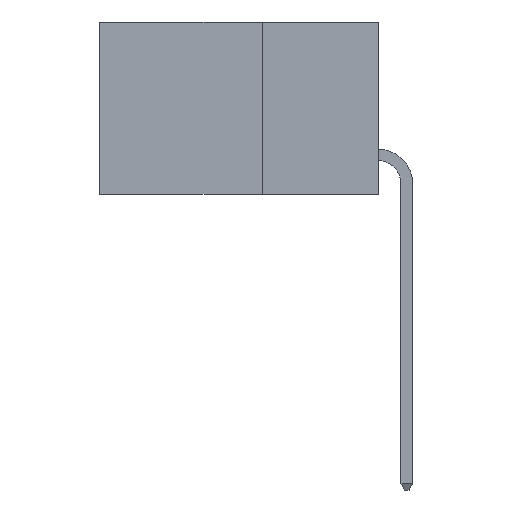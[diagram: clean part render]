
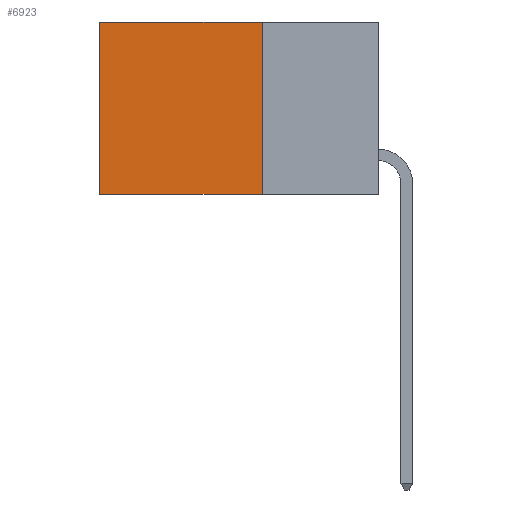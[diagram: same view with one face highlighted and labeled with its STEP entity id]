
A CAD part, left-side view. The second image highlights one B-rep face of the part: STEP entity #6923.
In plain terms, the highlighted planar face has unit normal (-1, 0, 0).
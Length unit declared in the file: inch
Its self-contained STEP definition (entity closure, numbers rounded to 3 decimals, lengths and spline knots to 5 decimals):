
#211 = CARTESIAN_POINT ( 'NONE',  ( 0.2615, 0.25, -0.37 ) ) ;
#429 = EDGE_CURVE ( 'NONE', #11617, #3420, #15281, .T. ) ;
#715 = DIRECTION ( 'NONE',  ( 0., 0., -1. ) ) ;
#1415 = EDGE_CURVE ( 'NONE', #8725, #10279, #13659, .T. ) ;
#1551 = DIRECTION ( 'NONE',  ( 0., 1., 0. ) ) ;
#1639 = DIRECTION ( 'NONE',  ( 0., 0., -1. ) ) ;
#2571 = DIRECTION ( 'NONE',  ( 0., 1., 0. ) ) ;
#2729 = EDGE_CURVE ( 'NONE', #11617, #8725, #12556, .T. ) ;
#2828 = ORIENTED_EDGE ( 'NONE', *, *, #9969, .F. ) ;
#2847 = CARTESIAN_POINT ( 'NONE',  ( 0.2615, 0.25, -0.37 ) ) ;
#3420 = VERTEX_POINT ( 'NONE', #211 ) ;
#4129 = ORIENTED_EDGE ( 'NONE', *, *, #1415, .T. ) ;
#4399 = CARTESIAN_POINT ( 'NONE',  ( 0.2615, 0.25, 0. ) ) ;
#4596 = CARTESIAN_POINT ( 'NONE',  ( 0.2615, 0.6, -0.37 ) ) ;
#4972 = LINE ( 'NONE', #2847, #14070 ) ;
#5332 = CARTESIAN_POINT ( 'NONE',  ( 0.2615, 0.25, -0.37 ) ) ;
#5451 = ORIENTED_EDGE ( 'NONE', *, *, #429, .F. ) ;
#6260 = CARTESIAN_POINT ( 'NONE',  ( 0.2615, 0.6, 0. ) ) ;
#6923 = ADVANCED_FACE ( 'NONE', ( #7392 ), #7849, .F. ) ;
#7073 = AXIS2_PLACEMENT_3D ( 'NONE', #5332, #9065, #1639 ) ;
#7392 = FACE_OUTER_BOUND ( 'NONE', #9972, .T. ) ;
#7445 = VECTOR ( 'NONE', #8824, 39.37008 ) ;
#7849 = PLANE ( 'NONE',  #7073 ) ;
#7953 = CARTESIAN_POINT ( 'NONE',  ( 0.2615, 0.25, -0.37 ) ) ;
#8632 = CARTESIAN_POINT ( 'NONE',  ( 0.2615, 0.6, -0.37 ) ) ;
#8725 = VERTEX_POINT ( 'NONE', #6260 ) ;
#8824 = DIRECTION ( 'NONE',  ( 0., 0., -1. ) ) ;
#9065 = DIRECTION ( 'NONE',  ( 1., 0., 0. ) ) ;
#9366 = ORIENTED_EDGE ( 'NONE', *, *, #2729, .T. ) ;
#9497 = VECTOR ( 'NONE', #2571, 39.37008 ) ;
#9969 = EDGE_CURVE ( 'NONE', #3420, #10279, #4972, .T. ) ;
#9972 = EDGE_LOOP ( 'NONE', ( #4129, #2828, #5451, #9366 ) ) ;
#10279 = VERTEX_POINT ( 'NONE', #4596 ) ;
#11617 = VERTEX_POINT ( 'NONE', #4399 ) ;
#11923 = VECTOR ( 'NONE', #715, 39.37008 ) ;
#12556 = LINE ( 'NONE', #13242, #9497 ) ;
#13242 = CARTESIAN_POINT ( 'NONE',  ( 0.2615, 0.25, 0. ) ) ;
#13659 = LINE ( 'NONE', #8632, #7445 ) ;
#14070 = VECTOR ( 'NONE', #1551, 39.37008 ) ;
#15281 = LINE ( 'NONE', #7953, #11923 ) ;
